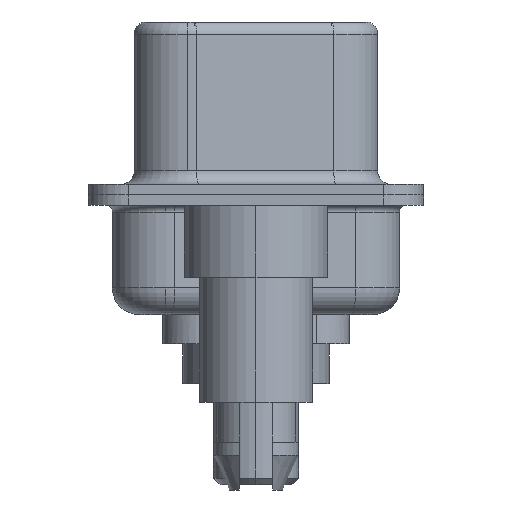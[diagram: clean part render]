
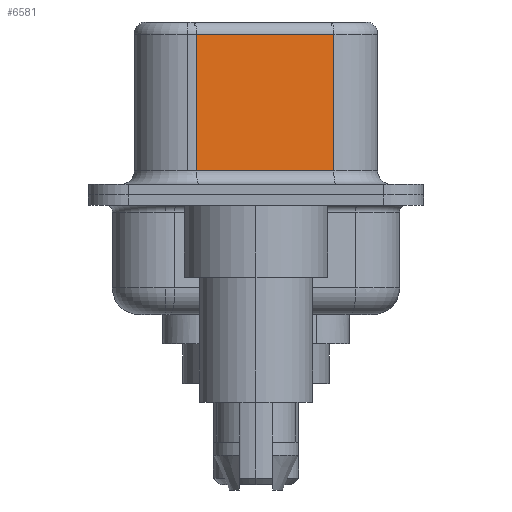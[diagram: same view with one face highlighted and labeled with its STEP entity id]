
A CAD part, left-side view. The second image highlights one B-rep face of the part: STEP entity #6581.
In plain terms, the highlighted planar face has unit normal (-0.985, -0.174, 0).
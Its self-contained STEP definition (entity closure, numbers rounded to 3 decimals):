
#1076 = VECTOR ( 'NONE', #7691, 1000. ) ;
#1232 = FACE_OUTER_BOUND ( 'NONE', #3877, .T. ) ;
#1576 = CARTESIAN_POINT ( 'NONE',  ( 3.67, 2.233, 6.02 ) ) ;
#2016 = VECTOR ( 'NONE', #11674, 1000. ) ;
#2359 = CARTESIAN_POINT ( 'NONE',  ( 4.58, -2.927, 0.9 ) ) ;
#2517 = DIRECTION ( 'NONE',  ( -0.174, 0.985, 0. ) ) ;
#3014 = EDGE_CURVE ( 'NONE', #3103, #7600, #14751, .T. ) ;
#3103 = VERTEX_POINT ( 'NONE', #1576 ) ;
#3405 = AXIS2_PLACEMENT_3D ( 'NONE', #14219, #11595, #2517 ) ;
#3645 = DIRECTION ( 'NONE',  ( -0.174, 0.985, 0. ) ) ;
#3877 = EDGE_LOOP ( 'NONE', ( #13519, #10449, #12593, #7253 ) ) ;
#3960 = CARTESIAN_POINT ( 'NONE',  ( 3.67, 2.233, 0.9 ) ) ;
#4429 = EDGE_CURVE ( 'NONE', #6137, #16164, #8906, .T. ) ;
#4837 = CARTESIAN_POINT ( 'NONE',  ( 4.58, -2.927, 6.02 ) ) ;
#5520 = LINE ( 'NONE', #2359, #2016 ) ;
#5718 = VECTOR ( 'NONE', #3645, 1000. ) ;
#6137 = VERTEX_POINT ( 'NONE', #8795 ) ;
#6581 = ADVANCED_FACE ( 'NONE', ( #1232 ), #7782, .F. ) ;
#7169 = EDGE_CURVE ( 'NONE', #6137, #3103, #13693, .T. ) ;
#7253 = ORIENTED_EDGE ( 'NONE', *, *, #14832, .T. ) ;
#7600 = VERTEX_POINT ( 'NONE', #3960 ) ;
#7691 = DIRECTION ( 'NONE',  ( 0., 0., -1. ) ) ;
#7782 = PLANE ( 'NONE',  #3405 ) ;
#8795 = CARTESIAN_POINT ( 'NONE',  ( 4.58, -2.927, 6.02 ) ) ;
#8906 = LINE ( 'NONE', #12834, #1076 ) ;
#10425 = CARTESIAN_POINT ( 'NONE',  ( 4.58, -2.927, 0.9 ) ) ;
#10449 = ORIENTED_EDGE ( 'NONE', *, *, #7169, .T. ) ;
#10830 = VECTOR ( 'NONE', #13002, 1000. ) ;
#11595 = DIRECTION ( 'NONE',  ( 0.985, 0.174, 0. ) ) ;
#11674 = DIRECTION ( 'NONE',  ( 0.174, -0.985, 0. ) ) ;
#12593 = ORIENTED_EDGE ( 'NONE', *, *, #3014, .T. ) ;
#12834 = CARTESIAN_POINT ( 'NONE',  ( 4.58, -2.927, 6.52 ) ) ;
#13002 = DIRECTION ( 'NONE',  ( 0., 0., -1. ) ) ;
#13519 = ORIENTED_EDGE ( 'NONE', *, *, #4429, .F. ) ;
#13693 = LINE ( 'NONE', #4837, #5718 ) ;
#14219 = CARTESIAN_POINT ( 'NONE',  ( 4.58, -2.927, 6.52 ) ) ;
#14249 = CARTESIAN_POINT ( 'NONE',  ( 3.67, 2.233, 6.52 ) ) ;
#14751 = LINE ( 'NONE', #14249, #10830 ) ;
#14832 = EDGE_CURVE ( 'NONE', #7600, #16164, #5520, .T. ) ;
#16164 = VERTEX_POINT ( 'NONE', #10425 ) ;
